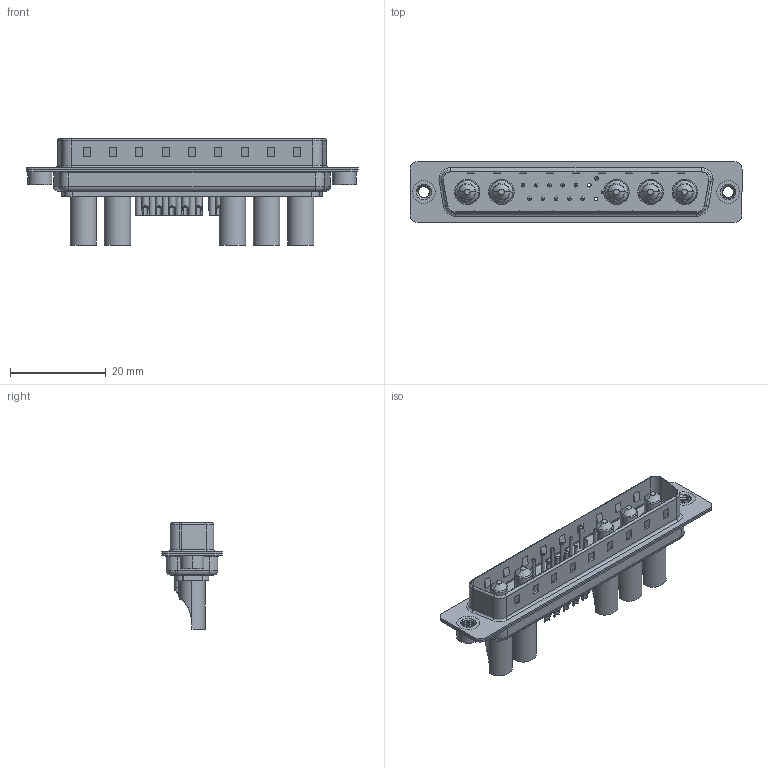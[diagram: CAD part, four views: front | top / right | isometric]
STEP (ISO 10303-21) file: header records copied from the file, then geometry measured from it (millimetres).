
FILE_DESCRIPTION (( 'STEP AP203' ), '1' );
FILE_NAME ('627-17W5222-4NA.STEP', '2019-05-29T01:05:17', ( '' ), ( '' ), 'SwSTEP 2.0', 'SolidWorks 2016', '' );
FILE_SCHEMA (( 'CONFIG_CONTROL_DESIGN' ));
Length unit declared in the file: millimetre
Products named in the file (9): 627Combo Contact Row 2_22; 627-17W5222-4NA; 627Combo Housing_17W5; 627Combo Shell Rear_37 Contacts; 627Combo Shell Front_37 Contacts; 627Combo Threaded Rivet_A; Power Pin_40A SC; 627Combo Threaded Rivet_2; 627Combo Contact Row 1_22
Assembly tree (22 placements, depth 2):
  627-17W5222-4NA
    627Combo Housing_17W5
    627Combo Shell Rear_37 Contacts
    627Combo Shell Front_37 Contacts
    627Combo Threaded Rivet_A
    Power Pin_40A SC  x5
    627Combo Threaded Rivet_2
    627Combo Contact Row 1_22  x6
    627Combo Contact Row 2_22  x6
Bounding box: 69.3 x 12.6 x 22.3 mm (x, y, z)
Volume: 4330.1 mm3; surface area: 9897 mm2
Topology: 27 solids, 27 shells, 1070 faces, 2542 edges, 1561 vertices
Faces by surface type: cylinder 434, plane 371, torus 180, cone 69, bspline 16
Entity records: 23304 total; most frequent: CARTESIAN_POINT 6700, DIRECTION 3334, ORIENTED_EDGE 3076, EDGE_CURVE 1538, AXIS2_PLACEMENT_3D 1258, VERTEX_POINT 975, VECTOR 818, LINE 818
